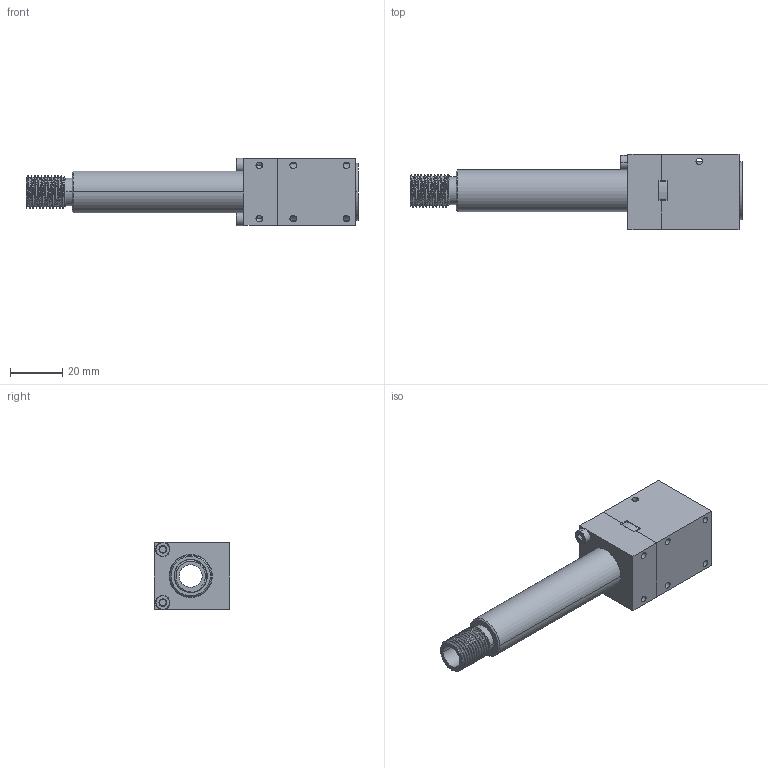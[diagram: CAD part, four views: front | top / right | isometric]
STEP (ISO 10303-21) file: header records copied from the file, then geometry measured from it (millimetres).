
FILE_DESCRIPTION (( 'STEP AP214' ), '1' );
FILE_NAME ('PPDW9 V4 wildcat barrel and block.STEP', '2020-12-31T18:27:18', ( '' ), ( '' ), 'SwSTEP 2.0', 'SolidWorks 2020', '' );
FILE_SCHEMA (( 'AUTOMOTIVE_DESIGN' ));
Length unit declared in the file: inch
Products named in the file (5): PPDW9 V4 wildcat barrel block; PPDW9 V4 wildcat barrel and block; PPDW9 V4 wildcat barrel block clamp; M3 x 25mm SHCS 91290A125_BLACK_91290A125; Barrel PPDW9 V2
Assembly tree (5 placements, depth 2):
  PPDW9 V4 wildcat barrel and block
    Barrel PPDW9 V2
    PPDW9 V4 wildcat barrel block
    PPDW9 V4 wildcat barrel block clamp
    M3 x 25mm SHCS 91290A125_BLACK_91290A125  x2
Bounding box: 126.82 x 28.7 x 25.82 mm (x, y, z)
Volume: 37713.4 mm3; surface area: 22487.2 mm2
Topology: 5 solids, 5 shells, 566 faces, 1581 edges, 1033 vertices
Faces by surface type: cylinder 371, plane 95, cone 61, bspline 35, torus 4
Entity records: 23398 total; most frequent: CARTESIAN_POINT 14093, ORIENTED_EDGE 2148, DIRECTION 1501, EDGE_CURVE 1074, VERTEX_POINT 707, AXIS2_PLACEMENT_3D 522, LINE 457, VECTOR 457
